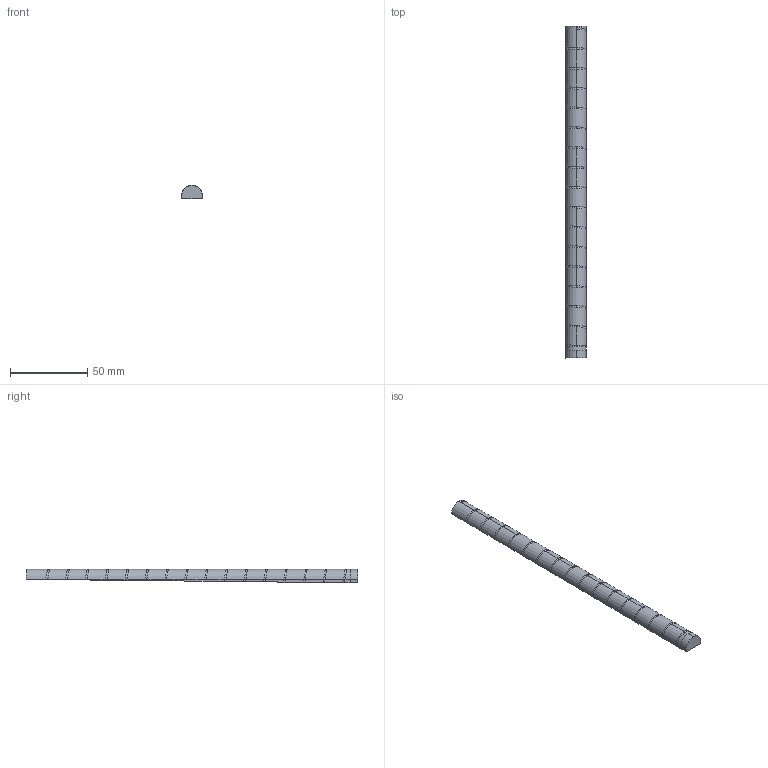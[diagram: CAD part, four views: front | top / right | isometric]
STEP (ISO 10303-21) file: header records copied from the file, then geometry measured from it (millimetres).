
FILE_DESCRIPTION(/* description */ (''),/* implementation_level */ '2;1');
FILE_NAME(/* name */ 'Side section 2.stp',/* time_stamp */ '2018-12-05T17:40:44-06:00',/* author */ ('johne'),/* organization */ (''),/* preprocessor_version */ 'ST-DEVELOPER v16.13',/* originating_system */ 'Autodesk Inventor 2018',/* authorisation */ '');
FILE_SCHEMA (('AUTOMOTIVE_DESIGN { 1 0 10303 214 3 1 1 }'));
Length unit declared in the file: millimetre
Products named in the file (1): Side section 2
Bounding box: 13.53 x 214.55 x 8.86 mm (x, y, z)
Volume: 17521.8 mm3; surface area: 7945.8 mm2
Topology: 1 solids, 1 shells, 158 faces, 448 edges, 292 vertices
Faces by surface type: bspline 66, plane 56, cone 34, cylinder 2
Entity records: 8697 total; most frequent: CARTESIAN_POINT 4817, ORIENTED_EDGE 896, DIRECTION 717, EDGE_CURVE 448, VERTEX_POINT 292, AXIS2_PLACEMENT_3D 247, LINE 223, VECTOR 223
